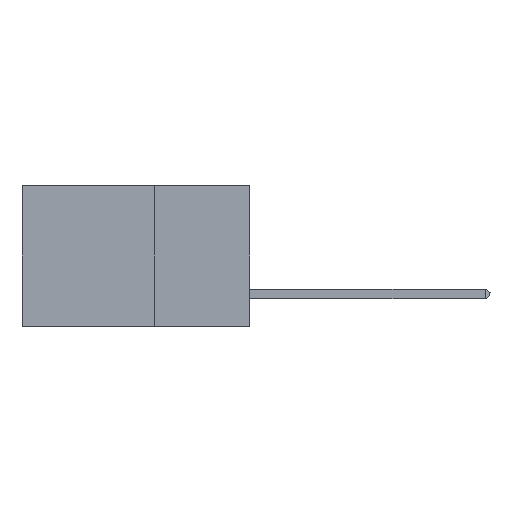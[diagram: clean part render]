
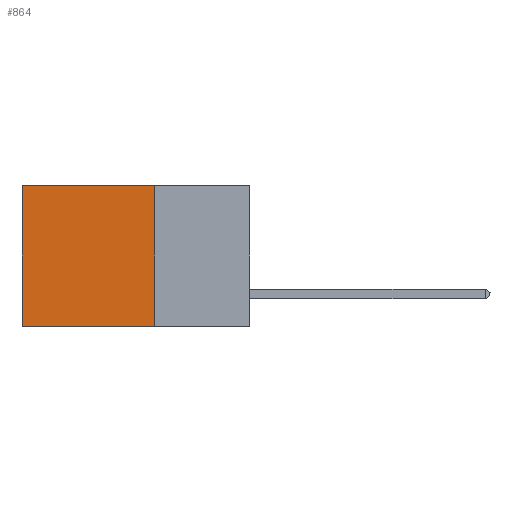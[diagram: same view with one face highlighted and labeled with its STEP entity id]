
A CAD part, left-side view. The second image highlights one B-rep face of the part: STEP entity #864.
In plain terms, the highlighted planar face has unit normal (-1, 0, 0).
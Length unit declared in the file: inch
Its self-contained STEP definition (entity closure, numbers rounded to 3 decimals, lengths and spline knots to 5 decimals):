
#481 = CARTESIAN_POINT ( 'NONE',  ( 0.2875, 0.25, 0. ) ) ;
#680 = DIRECTION ( 'NONE',  ( 0., 1., 0. ) ) ;
#864 = ADVANCED_FACE ( 'NONE', ( #34044 ), #10045, .F. ) ;
#1098 = LINE ( 'NONE', #7028, #3299 ) ;
#2855 = CARTESIAN_POINT ( 'NONE',  ( 0.2875, 0.25, -0.37 ) ) ;
#3299 = VECTOR ( 'NONE', #6879, 39.37008 ) ;
#3436 = VECTOR ( 'NONE', #14755, 39.37008 ) ;
#3981 = LINE ( 'NONE', #481, #3436 ) ;
#4827 = EDGE_CURVE ( 'NONE', #25801, #8308, #44566, .T. ) ;
#6639 = DIRECTION ( 'NONE',  ( 1., 0., 0. ) ) ;
#6879 = DIRECTION ( 'NONE',  ( 0., 1., 0. ) ) ;
#7028 = CARTESIAN_POINT ( 'NONE',  ( 0.2875, 0.25, 0. ) ) ;
#7548 = VERTEX_POINT ( 'NONE', #8114 ) ;
#8112 = EDGE_CURVE ( 'NONE', #11187, #7548, #1098, .T. ) ;
#8114 = CARTESIAN_POINT ( 'NONE',  ( 0.2875, 0.6, 0. ) ) ;
#8206 = AXIS2_PLACEMENT_3D ( 'NONE', #41973, #6639, #31404 ) ;
#8308 = VERTEX_POINT ( 'NONE', #23678 ) ;
#9517 = DIRECTION ( 'NONE',  ( 0., 0., -1. ) ) ;
#10045 = PLANE ( 'NONE',  #8206 ) ;
#10742 = ORIENTED_EDGE ( 'NONE', *, *, #43055, .T. ) ;
#11187 = VERTEX_POINT ( 'NONE', #37463 ) ;
#11775 = LINE ( 'NONE', #30703, #34017 ) ;
#11834 = ORIENTED_EDGE ( 'NONE', *, *, #37130, .F. ) ;
#13158 = EDGE_LOOP ( 'NONE', ( #10742, #40115, #11834, #30554 ) ) ;
#14755 = DIRECTION ( 'NONE',  ( 0., 0., -1. ) ) ;
#23678 = CARTESIAN_POINT ( 'NONE',  ( 0.2875, 0.6, -0.37 ) ) ;
#25801 = VERTEX_POINT ( 'NONE', #2855 ) ;
#30554 = ORIENTED_EDGE ( 'NONE', *, *, #8112, .T. ) ;
#30703 = CARTESIAN_POINT ( 'NONE',  ( 0.2875, 0.6, 0. ) ) ;
#31404 = DIRECTION ( 'NONE',  ( 0., 0., -1. ) ) ;
#34017 = VECTOR ( 'NONE', #9517, 39.37008 ) ;
#34044 = FACE_OUTER_BOUND ( 'NONE', #13158, .T. ) ;
#35699 = CARTESIAN_POINT ( 'NONE',  ( 0.2875, 0.25, -0.37 ) ) ;
#37130 = EDGE_CURVE ( 'NONE', #11187, #25801, #3981, .T. ) ;
#37463 = CARTESIAN_POINT ( 'NONE',  ( 0.2875, 0.25, 0. ) ) ;
#40115 = ORIENTED_EDGE ( 'NONE', *, *, #4827, .F. ) ;
#41973 = CARTESIAN_POINT ( 'NONE',  ( 0.2875, 0.25, 0. ) ) ;
#42918 = VECTOR ( 'NONE', #680, 39.37008 ) ;
#43055 = EDGE_CURVE ( 'NONE', #7548, #8308, #11775, .T. ) ;
#44566 = LINE ( 'NONE', #35699, #42918 ) ;
